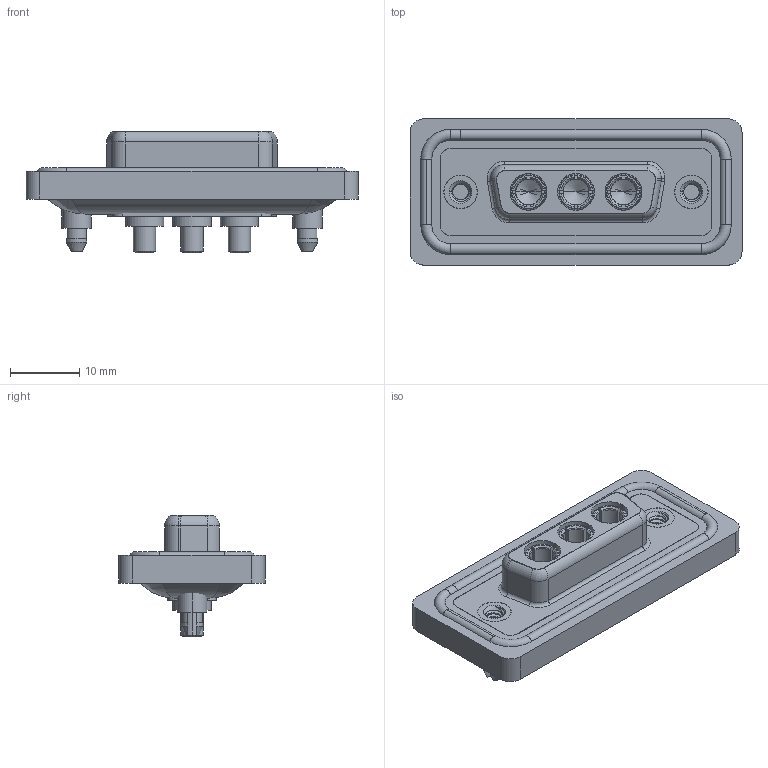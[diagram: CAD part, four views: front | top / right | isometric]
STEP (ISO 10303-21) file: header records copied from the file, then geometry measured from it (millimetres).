
FILE_DESCRIPTION (( 'STEP AP203' ), '1' );
FILE_NAME ('628W3W3-624-3N5.STEP', '2024-03-22T15:07:08', ( '' ), ( '' ), 'SwSTEP 2.0', 'SolidWorks 2023', '' );
FILE_SCHEMA (( 'CONFIG_CONTROL_DESIGN' ));
Length unit declared in the file: millimetre
Products named in the file (7): 628W3W3-624-3N5; 628Combo Housing_3W3; 628Combo Threaded Boardlock_5; 628Combo Shell Front_15 Contacts; 628Combo Shell Rear_15 Contacts; 628Combo Waterproof Housing_15 Contacts; Power Socket_30A S
Assembly tree (9 placements, depth 2):
  628W3W3-624-3N5
    628Combo Housing_3W3
    628Combo Waterproof Housing_15 Contacts
    628Combo Shell Front_15 Contacts
    628Combo Shell Rear_15 Contacts
    628Combo Threaded Boardlock_5  x2
    Power Socket_30A S  x3
Bounding box: 47.9 x 21.1 x 17.55 mm (x, y, z)
Volume: 6181.3 mm3; surface area: 10085.4 mm2
Topology: 13 solids, 13 shells, 658 faces, 1677 edges, 1065 vertices
Faces by surface type: cylinder 289, plane 208, torus 83, cone 65, bspline 13
Entity records: 16773 total; most frequent: CARTESIAN_POINT 4820, DIRECTION 2425, ORIENTED_EDGE 2304, EDGE_CURVE 1152, AXIS2_PLACEMENT_3D 965, VERTEX_POINT 732, EDGE_LOOP 508, CIRCLE 499
